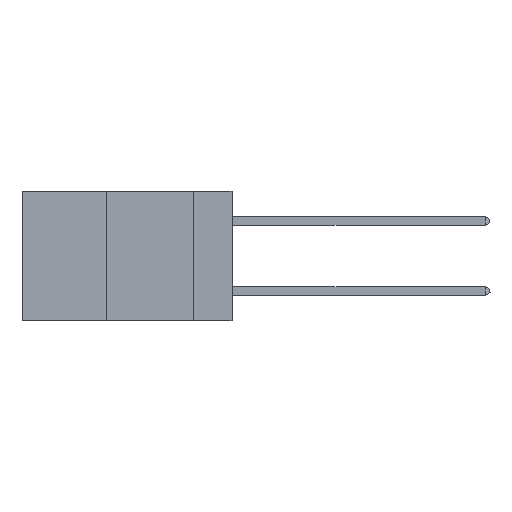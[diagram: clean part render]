
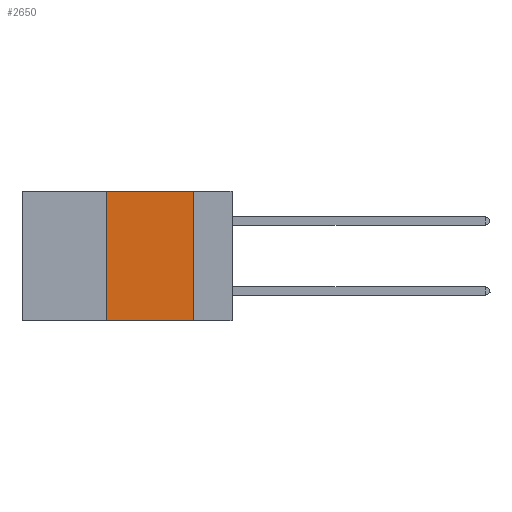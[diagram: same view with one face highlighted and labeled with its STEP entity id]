
A CAD part, left-side view. The second image highlights one B-rep face of the part: STEP entity #2650.
In plain terms, the highlighted planar face has unit normal (-1, 0, 0).
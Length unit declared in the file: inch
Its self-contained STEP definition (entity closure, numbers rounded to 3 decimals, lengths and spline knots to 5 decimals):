
#2650 = ADVANCED_FACE ( 'NONE', ( #13503 ), #26063, .F. ) ;
#3568 = EDGE_CURVE ( 'NONE', #12946, #7622, #6395, .T. ) ;
#3877 = LINE ( 'NONE', #28796, #12500 ) ;
#5777 = DIRECTION ( 'NONE',  ( 0., -1., 0. ) ) ;
#6395 = LINE ( 'NONE', #17620, #8877 ) ;
#6573 = DIRECTION ( 'NONE',  ( 0., 0., 1. ) ) ;
#6694 = EDGE_LOOP ( 'NONE', ( #17850, #10440, #13980, #17066 ) ) ;
#6908 = DIRECTION ( 'NONE',  ( 0., 0., -1. ) ) ;
#7237 = VECTOR ( 'NONE', #6573, 39.37008 ) ;
#7622 = VERTEX_POINT ( 'NONE', #12955 ) ;
#7962 = DIRECTION ( 'NONE',  ( 1., 0., 0. ) ) ;
#8877 = VECTOR ( 'NONE', #6908, 39.37008 ) ;
#9954 = EDGE_CURVE ( 'NONE', #11161, #20379, #25483, .T. ) ;
#10440 = ORIENTED_EDGE ( 'NONE', *, *, #19000, .F. ) ;
#11161 = VERTEX_POINT ( 'NONE', #24330 ) ;
#11314 = CARTESIAN_POINT ( 'NONE',  ( 0., 0.11, 0. ) ) ;
#12500 = VECTOR ( 'NONE', #5777, 39.37008 ) ;
#12578 = DIRECTION ( 'NONE',  ( 0., 0., -1. ) ) ;
#12665 = CARTESIAN_POINT ( 'NONE',  ( 0., 0.36, 0. ) ) ;
#12946 = VERTEX_POINT ( 'NONE', #11314 ) ;
#12955 = CARTESIAN_POINT ( 'NONE',  ( 0., 0.11, -0.37 ) ) ;
#12989 = AXIS2_PLACEMENT_3D ( 'NONE', #23501, #7962, #12578 ) ;
#13503 = FACE_OUTER_BOUND ( 'NONE', #6694, .T. ) ;
#13980 = ORIENTED_EDGE ( 'NONE', *, *, #9954, .F. ) ;
#15209 = CARTESIAN_POINT ( 'NONE',  ( 0., 0.6, -0.37 ) ) ;
#17066 = ORIENTED_EDGE ( 'NONE', *, *, #20501, .T. ) ;
#17373 = DIRECTION ( 'NONE',  ( 0., -1., 0. ) ) ;
#17620 = CARTESIAN_POINT ( 'NONE',  ( 0., 0.11, 0. ) ) ;
#17850 = ORIENTED_EDGE ( 'NONE', *, *, #3568, .F. ) ;
#19000 = EDGE_CURVE ( 'NONE', #20379, #12946, #3877, .T. ) ;
#19210 = LINE ( 'NONE', #15209, #27245 ) ;
#20379 = VERTEX_POINT ( 'NONE', #12665 ) ;
#20501 = EDGE_CURVE ( 'NONE', #11161, #7622, #19210, .T. ) ;
#22180 = CARTESIAN_POINT ( 'NONE',  ( 0., 0.36, 0. ) ) ;
#23501 = CARTESIAN_POINT ( 'NONE',  ( 0., 0.6, 0. ) ) ;
#24330 = CARTESIAN_POINT ( 'NONE',  ( 0., 0.36, -0.37 ) ) ;
#25483 = LINE ( 'NONE', #22180, #7237 ) ;
#26063 = PLANE ( 'NONE',  #12989 ) ;
#27245 = VECTOR ( 'NONE', #17373, 39.37008 ) ;
#28796 = CARTESIAN_POINT ( 'NONE',  ( 0., 0.6, 0. ) ) ;
